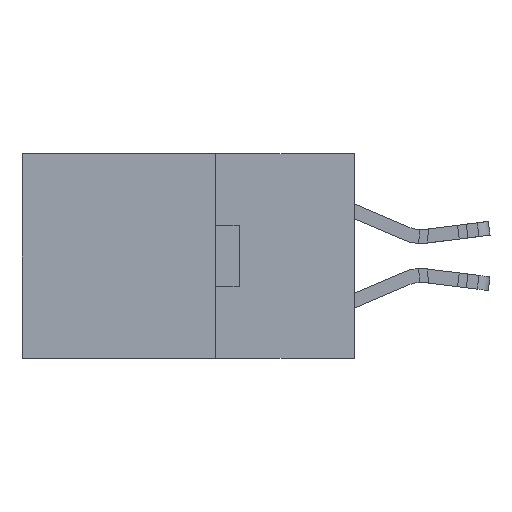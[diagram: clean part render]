
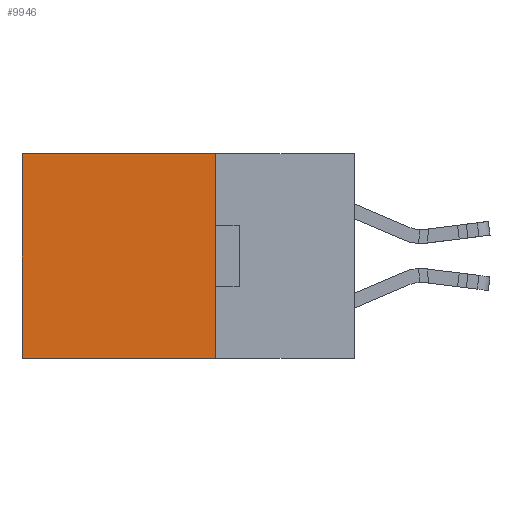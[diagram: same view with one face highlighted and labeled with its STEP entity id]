
A CAD part, left-side view. The second image highlights one B-rep face of the part: STEP entity #9946.
In plain terms, the highlighted planar face has unit normal (-1, 0, 0).
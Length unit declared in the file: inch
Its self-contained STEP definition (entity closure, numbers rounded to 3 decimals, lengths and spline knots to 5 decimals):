
#48 = CARTESIAN_POINT ( 'NONE',  ( 0.2615, 0.25, -0.37 ) ) ;
#256 = CARTESIAN_POINT ( 'NONE',  ( 0.2615, 0.25, -0.37 ) ) ;
#333 = ORIENTED_EDGE ( 'NONE', *, *, #22620, .F. ) ;
#1024 = CARTESIAN_POINT ( 'NONE',  ( 0.2615, 0.6, -0.37 ) ) ;
#1701 = VECTOR ( 'NONE', #25506, 39.37008 ) ;
#1983 = EDGE_CURVE ( 'NONE', #7545, #5592, #18784, .T. ) ;
#2221 = LINE ( 'NONE', #12991, #1701 ) ;
#3409 = AXIS2_PLACEMENT_3D ( 'NONE', #256, #6390, #10626 ) ;
#4743 = VECTOR ( 'NONE', #9684, 39.37008 ) ;
#5592 = VERTEX_POINT ( 'NONE', #18337 ) ;
#6138 = CARTESIAN_POINT ( 'NONE',  ( 0.2615, 0.6, -0.37 ) ) ;
#6166 = CARTESIAN_POINT ( 'NONE',  ( 0.2615, 0.25, 0. ) ) ;
#6317 = EDGE_LOOP ( 'NONE', ( #20884, #333, #25435, #20110 ) ) ;
#6390 = DIRECTION ( 'NONE',  ( 1., 0., 0. ) ) ;
#7049 = EDGE_CURVE ( 'NONE', #5592, #7081, #20462, .T. ) ;
#7081 = VERTEX_POINT ( 'NONE', #6138 ) ;
#7545 = VERTEX_POINT ( 'NONE', #6166 ) ;
#9042 = VECTOR ( 'NONE', #22835, 39.37008 ) ;
#9135 = VERTEX_POINT ( 'NONE', #48 ) ;
#9684 = DIRECTION ( 'NONE',  ( 0., 0., -1. ) ) ;
#9946 = ADVANCED_FACE ( 'NONE', ( #17720 ), #17575, .F. ) ;
#10626 = DIRECTION ( 'NONE',  ( 0., 0., -1. ) ) ;
#12991 = CARTESIAN_POINT ( 'NONE',  ( 0.2615, 0.25, -0.37 ) ) ;
#16768 = VECTOR ( 'NONE', #27466, 39.37008 ) ;
#17575 = PLANE ( 'NONE',  #3409 ) ;
#17720 = FACE_OUTER_BOUND ( 'NONE', #6317, .T. ) ;
#18023 = LINE ( 'NONE', #26704, #9042 ) ;
#18337 = CARTESIAN_POINT ( 'NONE',  ( 0.2615, 0.6, 0. ) ) ;
#18784 = LINE ( 'NONE', #27183, #16768 ) ;
#20110 = ORIENTED_EDGE ( 'NONE', *, *, #1983, .T. ) ;
#20462 = LINE ( 'NONE', #1024, #4743 ) ;
#20884 = ORIENTED_EDGE ( 'NONE', *, *, #7049, .T. ) ;
#22620 = EDGE_CURVE ( 'NONE', #9135, #7081, #2221, .T. ) ;
#22835 = DIRECTION ( 'NONE',  ( 0., 0., -1. ) ) ;
#25435 = ORIENTED_EDGE ( 'NONE', *, *, #27244, .F. ) ;
#25506 = DIRECTION ( 'NONE',  ( 0., 1., 0. ) ) ;
#26704 = CARTESIAN_POINT ( 'NONE',  ( 0.2615, 0.25, -0.37 ) ) ;
#27183 = CARTESIAN_POINT ( 'NONE',  ( 0.2615, 0.25, 0. ) ) ;
#27244 = EDGE_CURVE ( 'NONE', #7545, #9135, #18023, .T. ) ;
#27466 = DIRECTION ( 'NONE',  ( 0., 1., 0. ) ) ;
